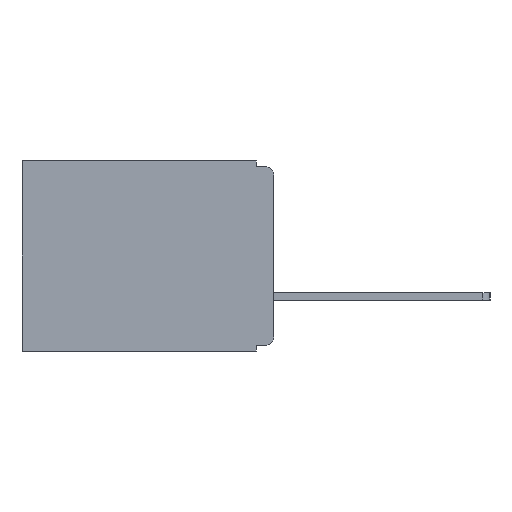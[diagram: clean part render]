
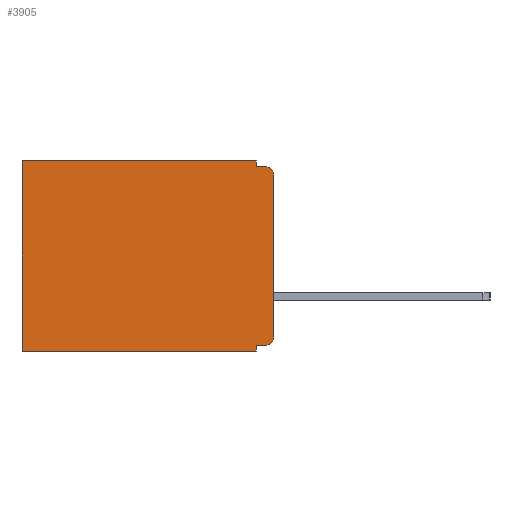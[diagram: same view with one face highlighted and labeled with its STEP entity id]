
A CAD part, left-side view. The second image highlights one B-rep face of the part: STEP entity #3905.
In plain terms, the highlighted planar face has unit normal (-1, 0, 0).
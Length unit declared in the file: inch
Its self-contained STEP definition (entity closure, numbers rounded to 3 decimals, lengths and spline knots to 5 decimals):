
#135 = LINE ( 'NONE', #19365, #13261 ) ;
#319 = VERTEX_POINT ( 'NONE', #11027 ) ;
#523 = LINE ( 'NONE', #11405, #3950 ) ;
#663 = DIRECTION ( 'NONE',  ( 0., 0., -1. ) ) ;
#711 = ORIENTED_EDGE ( 'NONE', *, *, #9872, .F. ) ;
#1149 = DIRECTION ( 'NONE',  ( 0., 1., 0. ) ) ;
#1331 = CARTESIAN_POINT ( 'NONE',  ( 0.3, 0., -0.32 ) ) ;
#1520 = VERTEX_POINT ( 'NONE', #18040 ) ;
#2281 = ORIENTED_EDGE ( 'NONE', *, *, #8523, .T. ) ;
#2752 = CARTESIAN_POINT ( 'NONE',  ( 0.3, 0.015, -0.025 ) ) ;
#3822 = EDGE_CURVE ( 'NONE', #13799, #5451, #5521, .T. ) ;
#3905 = ADVANCED_FACE ( 'NONE', ( #20971 ), #9845, .F. ) ;
#3932 = CIRCLE ( 'NONE', #21104, 0.015 ) ;
#3950 = VECTOR ( 'NONE', #1149, 39.37008 ) ;
#4421 = ORIENTED_EDGE ( 'NONE', *, *, #8973, .T. ) ;
#4446 = VECTOR ( 'NONE', #20633, 39.37008 ) ;
#4481 = DIRECTION ( 'NONE',  ( 0., 0., -1. ) ) ;
#5417 = EDGE_LOOP ( 'NONE', ( #711, #5742, #10871, #15421, #2281, #11419, #20952, #11972, #21465, #4421 ) ) ;
#5451 = VERTEX_POINT ( 'NONE', #6763 ) ;
#5521 = LINE ( 'NONE', #9943, #4446 ) ;
#5688 = EDGE_CURVE ( 'NONE', #7689, #5451, #12988, .T. ) ;
#5742 = ORIENTED_EDGE ( 'NONE', *, *, #11370, .T. ) ;
#6065 = DIRECTION ( 'NONE',  ( 0., 0., -1. ) ) ;
#6227 = CARTESIAN_POINT ( 'NONE',  ( 0.3, 0.031, -0.32 ) ) ;
#6763 = CARTESIAN_POINT ( 'NONE',  ( 0.3, 0.437, -0.33 ) ) ;
#6960 = VERTEX_POINT ( 'NONE', #9267 ) ;
#6977 = CARTESIAN_POINT ( 'NONE',  ( 0.3, 0.015, -0.01 ) ) ;
#7000 = EDGE_CURVE ( 'NONE', #18477, #8800, #21359, .T. ) ;
#7016 = AXIS2_PLACEMENT_3D ( 'NONE', #20985, #21970, #20246 ) ;
#7101 = CARTESIAN_POINT ( 'NONE',  ( 0.3, 0.031, -0.01 ) ) ;
#7689 = VERTEX_POINT ( 'NONE', #19296 ) ;
#8523 = EDGE_CURVE ( 'NONE', #12249, #13799, #523, .T. ) ;
#8705 = VECTOR ( 'NONE', #15233, 39.37008 ) ;
#8741 = CARTESIAN_POINT ( 'NONE',  ( 0.3, 0.031, 0. ) ) ;
#8800 = VERTEX_POINT ( 'NONE', #6977 ) ;
#8852 = CIRCLE ( 'NONE', #15379, 0.015 ) ;
#8973 = EDGE_CURVE ( 'NONE', #6960, #319, #3932, .T. ) ;
#9167 = CARTESIAN_POINT ( 'NONE',  ( 0.3, 0.015, -0.305 ) ) ;
#9267 = CARTESIAN_POINT ( 'NONE',  ( 0.3, 0.015, -0.32 ) ) ;
#9412 = DIRECTION ( 'NONE',  ( 0., -1., 0. ) ) ;
#9845 = PLANE ( 'NONE',  #7016 ) ;
#9872 = EDGE_CURVE ( 'NONE', #1520, #319, #13893, .T. ) ;
#9943 = CARTESIAN_POINT ( 'NONE',  ( 0.3, 0.437, -0.33 ) ) ;
#10871 = ORIENTED_EDGE ( 'NONE', *, *, #7000, .F. ) ;
#10933 = DIRECTION ( 'NONE',  ( 0., 0., -1. ) ) ;
#11027 = CARTESIAN_POINT ( 'NONE',  ( 0.3, 0., -0.305 ) ) ;
#11370 = EDGE_CURVE ( 'NONE', #1520, #8800, #8852, .T. ) ;
#11405 = CARTESIAN_POINT ( 'NONE',  ( 0.3, 0., 0. ) ) ;
#11419 = ORIENTED_EDGE ( 'NONE', *, *, #3822, .T. ) ;
#11972 = ORIENTED_EDGE ( 'NONE', *, *, #21467, .F. ) ;
#12188 = LINE ( 'NONE', #16342, #20640 ) ;
#12249 = VERTEX_POINT ( 'NONE', #8741 ) ;
#12448 = VECTOR ( 'NONE', #16075, 39.37008 ) ;
#12626 = EDGE_CURVE ( 'NONE', #6960, #13907, #15025, .T. ) ;
#12988 = LINE ( 'NONE', #14376, #12448 ) ;
#13261 = VECTOR ( 'NONE', #663, 39.37008 ) ;
#13537 = CARTESIAN_POINT ( 'NONE',  ( 0.3, 0., -0.33 ) ) ;
#13799 = VERTEX_POINT ( 'NONE', #17900 ) ;
#13893 = LINE ( 'NONE', #13537, #8705 ) ;
#13907 = VERTEX_POINT ( 'NONE', #6227 ) ;
#14376 = CARTESIAN_POINT ( 'NONE',  ( 0.3, 0., -0.33 ) ) ;
#14765 = DIRECTION ( 'NONE',  ( -1., 0., 0. ) ) ;
#15025 = LINE ( 'NONE', #1331, #18443 ) ;
#15233 = DIRECTION ( 'NONE',  ( 0., 0., -1. ) ) ;
#15379 = AXIS2_PLACEMENT_3D ( 'NONE', #2752, #14765, #4481 ) ;
#15421 = ORIENTED_EDGE ( 'NONE', *, *, #16125, .F. ) ;
#16075 = DIRECTION ( 'NONE',  ( 0., 1., 0. ) ) ;
#16125 = EDGE_CURVE ( 'NONE', #12249, #18477, #135, .T. ) ;
#16342 = CARTESIAN_POINT ( 'NONE',  ( 0.3, 0.031, -0.33 ) ) ;
#16887 = VECTOR ( 'NONE', #9412, 39.37008 ) ;
#17900 = CARTESIAN_POINT ( 'NONE',  ( 0.3, 0.437, 0. ) ) ;
#17920 = CARTESIAN_POINT ( 'NONE',  ( 0.3, 0., -0.01 ) ) ;
#18040 = CARTESIAN_POINT ( 'NONE',  ( 0.3, 0., -0.025 ) ) ;
#18443 = VECTOR ( 'NONE', #21765, 39.37008 ) ;
#18477 = VERTEX_POINT ( 'NONE', #7101 ) ;
#19296 = CARTESIAN_POINT ( 'NONE',  ( 0.3, 0.031, -0.33 ) ) ;
#19365 = CARTESIAN_POINT ( 'NONE',  ( 0.3, 0.031, 0. ) ) ;
#20246 = DIRECTION ( 'NONE',  ( 0., 0., -1. ) ) ;
#20633 = DIRECTION ( 'NONE',  ( 0., 0., -1. ) ) ;
#20640 = VECTOR ( 'NONE', #6065, 39.37008 ) ;
#20952 = ORIENTED_EDGE ( 'NONE', *, *, #5688, .F. ) ;
#20971 = FACE_OUTER_BOUND ( 'NONE', #5417, .T. ) ;
#20985 = CARTESIAN_POINT ( 'NONE',  ( 0.3, 0., -0.33 ) ) ;
#21082 = DIRECTION ( 'NONE',  ( -1., 0., 0. ) ) ;
#21104 = AXIS2_PLACEMENT_3D ( 'NONE', #9167, #21082, #10933 ) ;
#21359 = LINE ( 'NONE', #17920, #16887 ) ;
#21465 = ORIENTED_EDGE ( 'NONE', *, *, #12626, .F. ) ;
#21467 = EDGE_CURVE ( 'NONE', #13907, #7689, #12188, .T. ) ;
#21765 = DIRECTION ( 'NONE',  ( 0., 1., 0. ) ) ;
#21970 = DIRECTION ( 'NONE',  ( 1., 0., 0. ) ) ;
